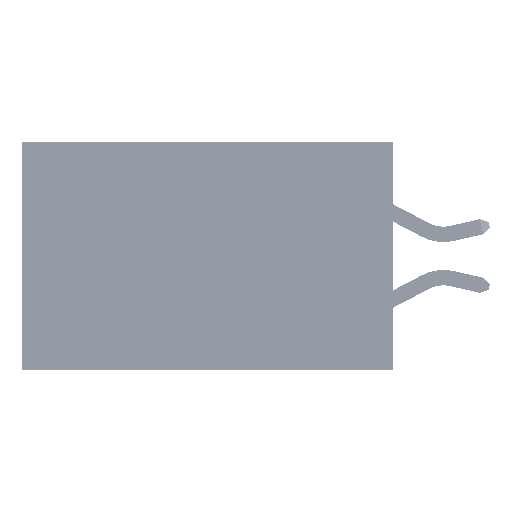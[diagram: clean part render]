
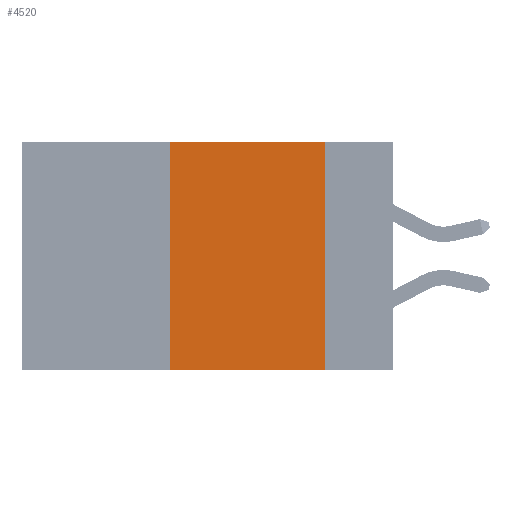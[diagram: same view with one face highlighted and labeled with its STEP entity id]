
A CAD part, left-side view. The second image highlights one B-rep face of the part: STEP entity #4520.
In plain terms, the highlighted planar face has unit normal (-1, 0, 0).
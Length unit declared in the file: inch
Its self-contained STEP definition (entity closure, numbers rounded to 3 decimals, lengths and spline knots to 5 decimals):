
#53 = VECTOR ( 'NONE', #37976, 39.37008 ) ;
#789 = EDGE_CURVE ( 'NONE', #29528, #19200, #16430, .T. ) ;
#903 = LINE ( 'NONE', #10010, #39924 ) ;
#1718 = DIRECTION ( 'NONE',  ( 0., 0., -1. ) ) ;
#1946 = ORIENTED_EDGE ( 'NONE', *, *, #5790, .T. ) ;
#2466 = EDGE_LOOP ( 'NONE', ( #10665, #15239, #18857, #1946 ) ) ;
#4520 = ADVANCED_FACE ( 'NONE', ( #14325 ), #39753, .F. ) ;
#5790 = EDGE_CURVE ( 'NONE', #6435, #14355, #22534, .T. ) ;
#6435 = VERTEX_POINT ( 'NONE', #47834 ) ;
#7653 = CARTESIAN_POINT ( 'NONE',  ( 0., 0.11, -0.37 ) ) ;
#8324 = LINE ( 'NONE', #34345, #53 ) ;
#9689 = AXIS2_PLACEMENT_3D ( 'NONE', #35278, #46966, #1718 ) ;
#10010 = CARTESIAN_POINT ( 'NONE',  ( 0., 0.11, 0. ) ) ;
#10133 = CARTESIAN_POINT ( 'NONE',  ( 0., 0.36, 0. ) ) ;
#10665 = ORIENTED_EDGE ( 'NONE', *, *, #30769, .F. ) ;
#13513 = DIRECTION ( 'NONE',  ( 0., 0., -1. ) ) ;
#14325 = FACE_OUTER_BOUND ( 'NONE', #2466, .T. ) ;
#14355 = VERTEX_POINT ( 'NONE', #7653 ) ;
#15034 = CARTESIAN_POINT ( 'NONE',  ( 0., 0.6, -0.37 ) ) ;
#15239 = ORIENTED_EDGE ( 'NONE', *, *, #789, .F. ) ;
#16430 = LINE ( 'NONE', #32449, #38296 ) ;
#18857 = ORIENTED_EDGE ( 'NONE', *, *, #35601, .F. ) ;
#19200 = VERTEX_POINT ( 'NONE', #23481 ) ;
#20210 = VECTOR ( 'NONE', #37339, 39.37008 ) ;
#21170 = DIRECTION ( 'NONE',  ( 0., -1., 0. ) ) ;
#22534 = LINE ( 'NONE', #15034, #20210 ) ;
#23481 = CARTESIAN_POINT ( 'NONE',  ( 0., 0.11, 0. ) ) ;
#29528 = VERTEX_POINT ( 'NONE', #10133 ) ;
#30769 = EDGE_CURVE ( 'NONE', #19200, #14355, #903, .T. ) ;
#32449 = CARTESIAN_POINT ( 'NONE',  ( 0., 0.6, 0. ) ) ;
#34345 = CARTESIAN_POINT ( 'NONE',  ( 0., 0.36, 0. ) ) ;
#35278 = CARTESIAN_POINT ( 'NONE',  ( 0., 0.6, 0. ) ) ;
#35601 = EDGE_CURVE ( 'NONE', #6435, #29528, #8324, .T. ) ;
#37339 = DIRECTION ( 'NONE',  ( 0., -1., 0. ) ) ;
#37976 = DIRECTION ( 'NONE',  ( 0., 0., 1. ) ) ;
#38296 = VECTOR ( 'NONE', #21170, 39.37008 ) ;
#39753 = PLANE ( 'NONE',  #9689 ) ;
#39924 = VECTOR ( 'NONE', #13513, 39.37008 ) ;
#46966 = DIRECTION ( 'NONE',  ( 1., 0., 0. ) ) ;
#47834 = CARTESIAN_POINT ( 'NONE',  ( 0., 0.36, -0.37 ) ) ;
